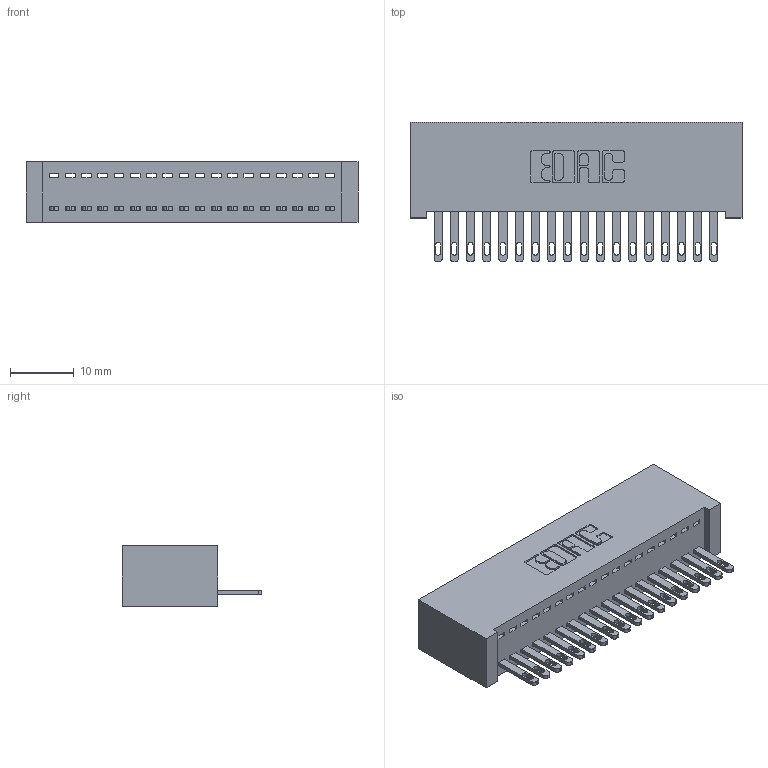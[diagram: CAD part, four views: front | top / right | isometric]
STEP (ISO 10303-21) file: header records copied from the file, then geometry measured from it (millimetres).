
FILE_DESCRIPTION (( 'STEP AP203' ), '1' );
FILE_NAME ('892-018-500-101.STEP', '2020-09-21T13:37:53', ( '' ), ( '' ), 'SwSTEP 2.0', 'SolidWorks 2020', '' );
FILE_SCHEMA (( 'CONFIG_CONTROL_DESIGN' ));
Length unit declared in the file: inch
Products named in the file (3): 892-018-500-101; 345-292-001_345-293-100; 842 Part_Lugless
Assembly tree (19 placements, depth 2):
  892-018-500-101
    842 Part_Lugless
    345-292-001_345-293-100  x18
Bounding box: 51.97 x 21.85 x 9.4 mm (x, y, z)
Volume: 4888.3 mm3; surface area: 7088.9 mm2
Topology: 19 solids, 19 shells, 1074 faces, 3299 edges, 2198 vertices
Faces by surface type: plane 710, cylinder 364
Entity records: 13629 total; most frequent: CARTESIAN_POINT 2360, ORIENTED_EDGE 2314, DIRECTION 2033, EDGE_CURVE 1157, LINE 1033, VECTOR 1033, VERTEX_POINT 770, AXIS2_PLACEMENT_3D 500
